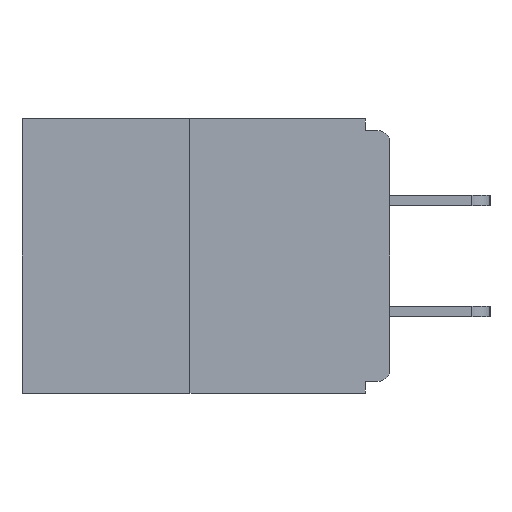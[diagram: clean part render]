
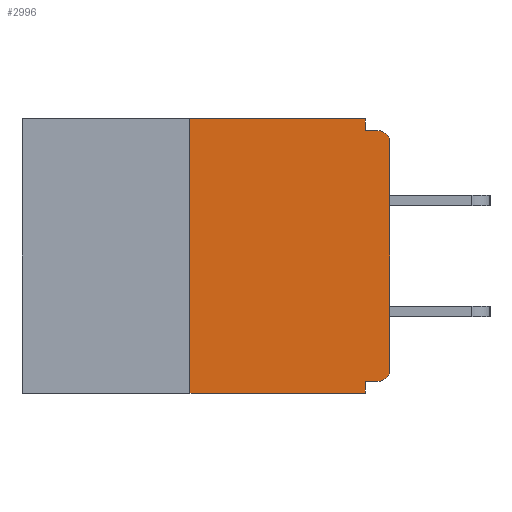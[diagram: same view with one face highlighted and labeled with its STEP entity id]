
A CAD part, left-side view. The second image highlights one B-rep face of the part: STEP entity #2996.
In plain terms, the highlighted planar face has unit normal (-1, 0, 0).
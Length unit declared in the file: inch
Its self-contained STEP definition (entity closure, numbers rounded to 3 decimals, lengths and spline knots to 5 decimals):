
#70 = EDGE_CURVE ( 'NONE', #10448, #9626, #4038, .T. ) ;
#116 = EDGE_LOOP ( 'NONE', ( #9215, #3170, #8403, #6225, #4608, #1876, #3731, #7080, #6244, #6584 ) ) ;
#134 = EDGE_CURVE ( 'NONE', #5077, #10840, #2517, .T. ) ;
#220 = DIRECTION ( 'NONE',  ( 0., 0., -1. ) ) ;
#291 = LINE ( 'NONE', #2902, #2478 ) ;
#426 = DIRECTION ( 'NONE',  ( 0., 0., 1. ) ) ;
#517 = DIRECTION ( 'NONE',  ( 0., -1., 0. ) ) ;
#1019 = LINE ( 'NONE', #1757, #1307 ) ;
#1135 = CARTESIAN_POINT ( 'NONE',  ( 0., 0.46, 0. ) ) ;
#1195 = VERTEX_POINT ( 'NONE', #9439 ) ;
#1230 = DIRECTION ( 'NONE',  ( 0., 0., -1. ) ) ;
#1273 = CARTESIAN_POINT ( 'NONE',  ( 0., 0., 0. ) ) ;
#1307 = VECTOR ( 'NONE', #4416, 39.37008 ) ;
#1757 = CARTESIAN_POINT ( 'NONE',  ( 0., 0.46, -0.343 ) ) ;
#1825 = CARTESIAN_POINT ( 'NONE',  ( 0., 0.25, 0. ) ) ;
#1876 = ORIENTED_EDGE ( 'NONE', *, *, #10257, .T. ) ;
#2038 = LINE ( 'NONE', #6162, #11142 ) ;
#2138 = VERTEX_POINT ( 'NONE', #9406 ) ;
#2478 = VECTOR ( 'NONE', #3229, 39.37008 ) ;
#2517 = LINE ( 'NONE', #4997, #7642 ) ;
#2533 = VECTOR ( 'NONE', #9873, 39.37008 ) ;
#2760 = VERTEX_POINT ( 'NONE', #3010 ) ;
#2767 = LINE ( 'NONE', #7952, #2533 ) ;
#2902 = CARTESIAN_POINT ( 'NONE',  ( 0., 0.031, -0.343 ) ) ;
#2996 = ADVANCED_FACE ( 'NONE', ( #7959 ), #6266, .F. ) ;
#3010 = CARTESIAN_POINT ( 'NONE',  ( 0., 0.25, -0.343 ) ) ;
#3170 = ORIENTED_EDGE ( 'NONE', *, *, #7114, .F. ) ;
#3171 = CARTESIAN_POINT ( 'NONE',  ( 0., 0., -0.313 ) ) ;
#3175 = VERTEX_POINT ( 'NONE', #1825 ) ;
#3214 = CIRCLE ( 'NONE', #3557, 0.015 ) ;
#3229 = DIRECTION ( 'NONE',  ( 0., 0., -1. ) ) ;
#3557 = AXIS2_PLACEMENT_3D ( 'NONE', #7789, #6045, #4411 ) ;
#3731 = ORIENTED_EDGE ( 'NONE', *, *, #70, .T. ) ;
#4038 = LINE ( 'NONE', #1273, #10745 ) ;
#4411 = DIRECTION ( 'NONE',  ( 0., 0., -1. ) ) ;
#4416 = DIRECTION ( 'NONE',  ( 0., -1., 0. ) ) ;
#4601 = DIRECTION ( 'NONE',  ( -1., 0., 0. ) ) ;
#4608 = ORIENTED_EDGE ( 'NONE', *, *, #134, .F. ) ;
#4790 = AXIS2_PLACEMENT_3D ( 'NONE', #10584, #9716, #220 ) ;
#4997 = CARTESIAN_POINT ( 'NONE',  ( 0., 0., -0.328 ) ) ;
#5055 = DIRECTION ( 'NONE',  ( 0., 1., 0. ) ) ;
#5077 = VERTEX_POINT ( 'NONE', #7820 ) ;
#5622 = VECTOR ( 'NONE', #517, 39.37008 ) ;
#5903 = AXIS2_PLACEMENT_3D ( 'NONE', #6233, #4601, #7125 ) ;
#6045 = DIRECTION ( 'NONE',  ( -1., 0., 0. ) ) ;
#6049 = LINE ( 'NONE', #1135, #10892 ) ;
#6162 = CARTESIAN_POINT ( 'NONE',  ( 0., 0.031, 0. ) ) ;
#6225 = ORIENTED_EDGE ( 'NONE', *, *, #10318, .F. ) ;
#6233 = CARTESIAN_POINT ( 'NONE',  ( 0., 0.015, -0.313 ) ) ;
#6244 = ORIENTED_EDGE ( 'NONE', *, *, #8010, .F. ) ;
#6266 = PLANE ( 'NONE',  #4790 ) ;
#6584 = ORIENTED_EDGE ( 'NONE', *, *, #9328, .F. ) ;
#6619 = CIRCLE ( 'NONE', #5903, 0.015 ) ;
#6702 = CARTESIAN_POINT ( 'NONE',  ( 0., 0.031, -0.328 ) ) ;
#7080 = ORIENTED_EDGE ( 'NONE', *, *, #9245, .T. ) ;
#7114 = EDGE_CURVE ( 'NONE', #2760, #3175, #2767, .T. ) ;
#7125 = DIRECTION ( 'NONE',  ( 0., 0., -1. ) ) ;
#7288 = LINE ( 'NONE', #10765, #5622 ) ;
#7523 = VERTEX_POINT ( 'NONE', #7936 ) ;
#7642 = VECTOR ( 'NONE', #5055, 39.37008 ) ;
#7789 = CARTESIAN_POINT ( 'NONE',  ( 0., 0.015, -0.03 ) ) ;
#7820 = CARTESIAN_POINT ( 'NONE',  ( 0., 0.015, -0.328 ) ) ;
#7936 = CARTESIAN_POINT ( 'NONE',  ( 0., 0.031, -0.343 ) ) ;
#7952 = CARTESIAN_POINT ( 'NONE',  ( 0., 0.25, 0. ) ) ;
#7959 = FACE_OUTER_BOUND ( 'NONE', #116, .T. ) ;
#8010 = EDGE_CURVE ( 'NONE', #2138, #1195, #7288, .T. ) ;
#8026 = VERTEX_POINT ( 'NONE', #10820 ) ;
#8344 = EDGE_CURVE ( 'NONE', #3175, #8026, #6049, .T. ) ;
#8370 = EDGE_CURVE ( 'NONE', #2760, #7523, #1019, .T. ) ;
#8403 = ORIENTED_EDGE ( 'NONE', *, *, #8370, .T. ) ;
#9033 = CARTESIAN_POINT ( 'NONE',  ( 0., 0., -0.03 ) ) ;
#9215 = ORIENTED_EDGE ( 'NONE', *, *, #8344, .F. ) ;
#9245 = EDGE_CURVE ( 'NONE', #9626, #1195, #3214, .T. ) ;
#9328 = EDGE_CURVE ( 'NONE', #8026, #2138, #2038, .T. ) ;
#9406 = CARTESIAN_POINT ( 'NONE',  ( 0., 0.031, -0.015 ) ) ;
#9439 = CARTESIAN_POINT ( 'NONE',  ( 0., 0.015, -0.015 ) ) ;
#9626 = VERTEX_POINT ( 'NONE', #9033 ) ;
#9716 = DIRECTION ( 'NONE',  ( 1., 0., 0. ) ) ;
#9873 = DIRECTION ( 'NONE',  ( 0., 0., 1. ) ) ;
#10257 = EDGE_CURVE ( 'NONE', #5077, #10448, #6619, .T. ) ;
#10318 = EDGE_CURVE ( 'NONE', #10840, #7523, #291, .T. ) ;
#10448 = VERTEX_POINT ( 'NONE', #3171 ) ;
#10544 = DIRECTION ( 'NONE',  ( 0., -1., 0. ) ) ;
#10584 = CARTESIAN_POINT ( 'NONE',  ( 0., 0.46, 0. ) ) ;
#10745 = VECTOR ( 'NONE', #426, 39.37008 ) ;
#10765 = CARTESIAN_POINT ( 'NONE',  ( 0., 0., -0.015 ) ) ;
#10820 = CARTESIAN_POINT ( 'NONE',  ( 0., 0.031, 0. ) ) ;
#10840 = VERTEX_POINT ( 'NONE', #6702 ) ;
#10892 = VECTOR ( 'NONE', #10544, 39.37008 ) ;
#11142 = VECTOR ( 'NONE', #1230, 39.37008 ) ;
